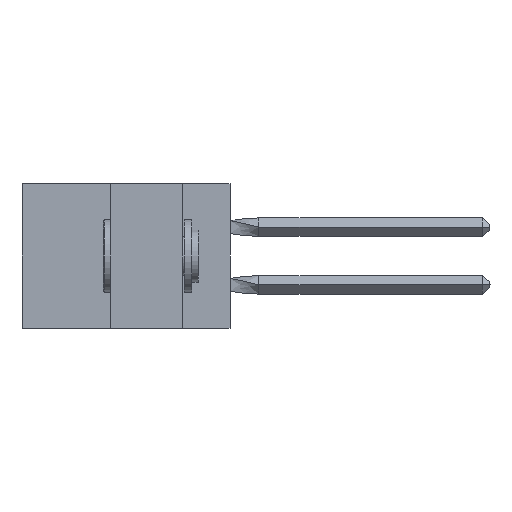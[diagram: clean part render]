
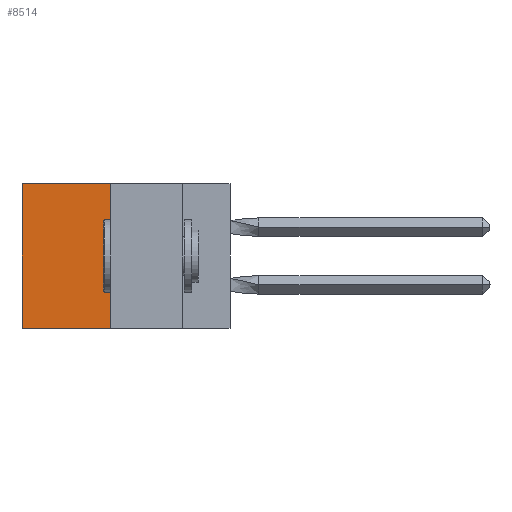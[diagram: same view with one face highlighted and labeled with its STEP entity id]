
A CAD part, left-side view. The second image highlights one B-rep face of the part: STEP entity #8514.
In plain terms, the highlighted planar face has unit normal (-1, 0, 0).
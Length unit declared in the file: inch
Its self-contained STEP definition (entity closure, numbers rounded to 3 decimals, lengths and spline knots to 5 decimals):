
#51 = CARTESIAN_POINT ( 'NONE',  ( 0.305, 0.72, -0.5 ) ) ;
#126 = CARTESIAN_POINT ( 'NONE',  ( 0.305, 0.413, -0.5 ) ) ;
#150 = LINE ( 'NONE', #1491, #13125 ) ;
#256 = DIRECTION ( 'NONE',  ( 0., 1., 0. ) ) ;
#293 = DIRECTION ( 'NONE',  ( 1., 0., 0. ) ) ;
#656 = ORIENTED_EDGE ( 'NONE', *, *, #9831, .F. ) ;
#715 = ORIENTED_EDGE ( 'NONE', *, *, #5096, .T. ) ;
#1465 = LINE ( 'NONE', #13751, #17769 ) ;
#1491 = CARTESIAN_POINT ( 'NONE',  ( 0.305, 0.413, 0. ) ) ;
#1600 = DIRECTION ( 'NONE',  ( 0., 0., -1. ) ) ;
#2270 = CARTESIAN_POINT ( 'NONE',  ( 0.305, 0.413, -0.5 ) ) ;
#4602 = CARTESIAN_POINT ( 'NONE',  ( 0.305, 0.413, -0.5 ) ) ;
#5096 = EDGE_CURVE ( 'NONE', #15643, #11755, #1465, .T. ) ;
#5827 = CARTESIAN_POINT ( 'NONE',  ( 0.305, 0.72, 0. ) ) ;
#8176 = CARTESIAN_POINT ( 'NONE',  ( 0.305, 0.413, 0. ) ) ;
#8383 = DIRECTION ( 'NONE',  ( 0., 0., -1. ) ) ;
#8438 = EDGE_CURVE ( 'NONE', #14188, #15643, #150, .T. ) ;
#8514 = ADVANCED_FACE ( 'NONE', ( #15489 ), #18282, .F. ) ;
#9334 = VECTOR ( 'NONE', #256, 39.37008 ) ;
#9424 = VERTEX_POINT ( 'NONE', #18431 ) ;
#9831 = EDGE_CURVE ( 'NONE', #14188, #9424, #11214, .T. ) ;
#10836 = AXIS2_PLACEMENT_3D ( 'NONE', #4602, #293, #18350 ) ;
#11092 = EDGE_CURVE ( 'NONE', #9424, #11755, #18334, .T. ) ;
#11214 = LINE ( 'NONE', #2270, #12412 ) ;
#11755 = VERTEX_POINT ( 'NONE', #51 ) ;
#12069 = DIRECTION ( 'NONE',  ( 0., 1., 0. ) ) ;
#12412 = VECTOR ( 'NONE', #8383, 39.37008 ) ;
#13125 = VECTOR ( 'NONE', #12069, 39.37008 ) ;
#13751 = CARTESIAN_POINT ( 'NONE',  ( 0.305, 0.72, -0.5 ) ) ;
#14164 = ORIENTED_EDGE ( 'NONE', *, *, #11092, .F. ) ;
#14188 = VERTEX_POINT ( 'NONE', #8176 ) ;
#14787 = EDGE_LOOP ( 'NONE', ( #715, #14164, #656, #19392 ) ) ;
#15489 = FACE_OUTER_BOUND ( 'NONE', #14787, .T. ) ;
#15643 = VERTEX_POINT ( 'NONE', #5827 ) ;
#17769 = VECTOR ( 'NONE', #1600, 39.37008 ) ;
#18282 = PLANE ( 'NONE',  #10836 ) ;
#18334 = LINE ( 'NONE', #126, #9334 ) ;
#18350 = DIRECTION ( 'NONE',  ( 0., 0., -1. ) ) ;
#18431 = CARTESIAN_POINT ( 'NONE',  ( 0.305, 0.413, -0.5 ) ) ;
#19392 = ORIENTED_EDGE ( 'NONE', *, *, #8438, .T. ) ;
